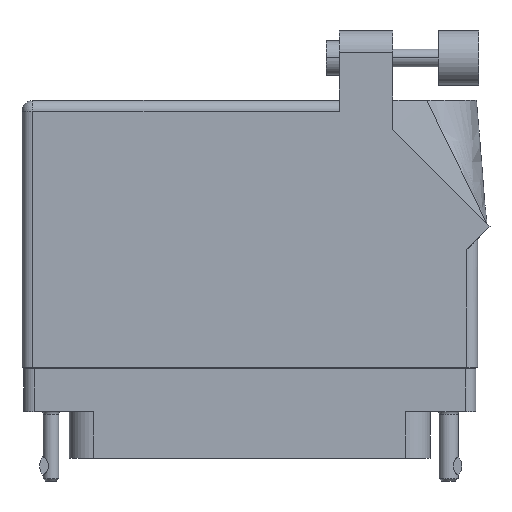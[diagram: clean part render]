
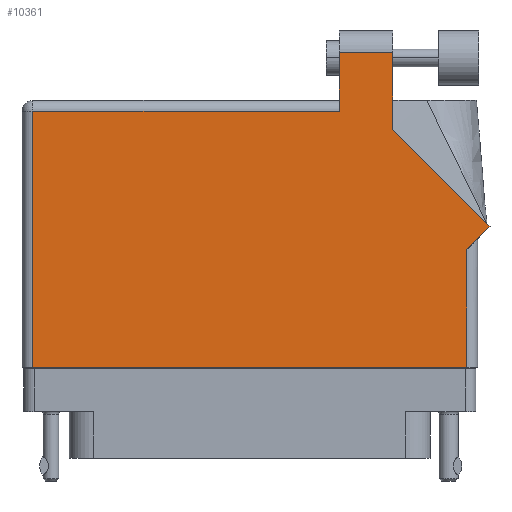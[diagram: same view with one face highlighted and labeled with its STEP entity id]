
A CAD part, front view. The second image highlights one B-rep face of the part: STEP entity #10361.
In plain terms, the highlighted face is planar.
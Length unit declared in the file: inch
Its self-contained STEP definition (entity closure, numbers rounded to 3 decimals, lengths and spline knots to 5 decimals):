
#507 = DIRECTION ( 'NONE',  ( 0., 1., 0. ) ) ;
#3400 = CARTESIAN_POINT ( 'NONE',  ( 1.306, 0.637, 0.455 ) ) ;
#3542 = VERTEX_POINT ( 'NONE', #5887 ) ;
#3811 = ORIENTED_EDGE ( 'NONE', *, *, #17329, .T. ) ;
#4860 = VECTOR ( 'NONE', #46146, 39.37008 ) ;
#5770 = ORIENTED_EDGE ( 'NONE', *, *, #61104, .T. ) ;
#5887 = CARTESIAN_POINT ( 'NONE',  ( 1.37671, 0.70771, 0.455 ) ) ;
#7554 = DIRECTION ( 'NONE',  ( 0., 0., -1. ) ) ;
#8658 = EDGE_LOOP ( 'NONE', ( #59539, #56673, #15471, #14280, #3811, #14995, #5770, #11784, #46687 ) ) ;
#10133 = LINE ( 'NONE', #57187, #55850 ) ;
#10361 = ADVANCED_FACE ( 'NONE', ( #16559 ), #35436, .F. ) ;
#11784 = ORIENTED_EDGE ( 'NONE', *, *, #49289, .T. ) ;
#14280 = ORIENTED_EDGE ( 'NONE', *, *, #25495, .T. ) ;
#14977 = AXIS2_PLACEMENT_3D ( 'NONE', #21819, #7554, #22240 ) ;
#14995 = ORIENTED_EDGE ( 'NONE', *, *, #37256, .T. ) ;
#15471 = ORIENTED_EDGE ( 'NONE', *, *, #34756, .T. ) ;
#16348 = DIRECTION ( 'NONE',  ( 1., 0., 0. ) ) ;
#16489 = VECTOR ( 'NONE', #59213, 39.37008 ) ;
#16559 = FACE_OUTER_BOUND ( 'NONE', #8658, .T. ) ;
#16572 = LINE ( 'NONE', #45083, #37260 ) ;
#16948 = CARTESIAN_POINT ( 'NONE',  ( 0.513, 1.705, 0.455 ) ) ;
#17329 = EDGE_CURVE ( 'NONE', #31396, #21033, #19677, .T. ) ;
#19677 = LINE ( 'NONE', #25045, #28486 ) ;
#21033 = VERTEX_POINT ( 'NONE', #59334 ) ;
#21819 = CARTESIAN_POINT ( 'NONE',  ( -1.306, 1.43, 0.455 ) ) ;
#21882 = VERTEX_POINT ( 'NONE', #48684 ) ;
#22240 = DIRECTION ( 'NONE',  ( -1., 0., 0. ) ) ;
#23289 = VERTEX_POINT ( 'NONE', #16948 ) ;
#23631 = EDGE_CURVE ( 'NONE', #3542, #53780, #16572, .T. ) ;
#25045 = CARTESIAN_POINT ( 'NONE',  ( -1.244, -0.1, 0.455 ) ) ;
#25495 = EDGE_CURVE ( 'NONE', #28730, #31396, #47323, .T. ) ;
#25578 = DIRECTION ( 'NONE',  ( -1., 0., 0. ) ) ;
#25584 = CARTESIAN_POINT ( 'NONE',  ( 0.513, 1.368, 0.455 ) ) ;
#26626 = LINE ( 'NONE', #34705, #42022 ) ;
#27619 = VERTEX_POINT ( 'NONE', #56955 ) ;
#28486 = VECTOR ( 'NONE', #39075, 39.37008 ) ;
#28730 = VERTEX_POINT ( 'NONE', #25584 ) ;
#30913 = LINE ( 'NONE', #33974, #35332 ) ;
#31396 = VERTEX_POINT ( 'NONE', #58039 ) ;
#33974 = CARTESIAN_POINT ( 'NONE',  ( 1.244, 0.637, 0.455 ) ) ;
#33987 = VERTEX_POINT ( 'NONE', #48193 ) ;
#34705 = CARTESIAN_POINT ( 'NONE',  ( -1.306, -0.1, 0.455 ) ) ;
#34756 = EDGE_CURVE ( 'NONE', #23289, #28730, #57760, .T. ) ;
#35332 = VECTOR ( 'NONE', #52729, 39.37008 ) ;
#35436 = PLANE ( 'NONE',  #14977 ) ;
#37256 = EDGE_CURVE ( 'NONE', #21033, #33987, #26626, .T. ) ;
#37260 = VECTOR ( 'NONE', #49786, 39.37008 ) ;
#39075 = DIRECTION ( 'NONE',  ( 0., -1., 0. ) ) ;
#40705 = VECTOR ( 'NONE', #25578, 39.37008 ) ;
#40854 = CARTESIAN_POINT ( 'NONE',  ( 0.513, 1.43, 0.455 ) ) ;
#41080 = CARTESIAN_POINT ( 'NONE',  ( 0.513, 1.705, 0.455 ) ) ;
#42022 = VECTOR ( 'NONE', #16348, 39.37008 ) ;
#45083 = CARTESIAN_POINT ( 'NONE',  ( 1.37671, 0.70771, 0.455 ) ) ;
#45819 = DIRECTION ( 'NONE',  ( -1., 0., 0. ) ) ;
#46146 = DIRECTION ( 'NONE',  ( 0.707, 0.707, 0. ) ) ;
#46687 = ORIENTED_EDGE ( 'NONE', *, *, #23631, .T. ) ;
#46973 = VECTOR ( 'NONE', #45819, 39.37008 ) ;
#47036 = LINE ( 'NONE', #41080, #46973 ) ;
#47323 = LINE ( 'NONE', #54361, #40705 ) ;
#48193 = CARTESIAN_POINT ( 'NONE',  ( 1.244, -0.1, 0.455 ) ) ;
#48612 = EDGE_CURVE ( 'NONE', #53780, #27619, #10133, .T. ) ;
#48684 = CARTESIAN_POINT ( 'NONE',  ( 1.244, 0.575, 0.455 ) ) ;
#49289 = EDGE_CURVE ( 'NONE', #21882, #3542, #50600, .T. ) ;
#49786 = DIRECTION ( 'NONE',  ( -0.707, 0.707, 0. ) ) ;
#50073 = CARTESIAN_POINT ( 'NONE',  ( 0.82, 1.26442, 0.455 ) ) ;
#50600 = LINE ( 'NONE', #3400, #4860 ) ;
#52729 = DIRECTION ( 'NONE',  ( 0., 1., 0. ) ) ;
#53780 = VERTEX_POINT ( 'NONE', #50073 ) ;
#54361 = CARTESIAN_POINT ( 'NONE',  ( -1.306, 1.368, 0.455 ) ) ;
#55850 = VECTOR ( 'NONE', #507, 39.37008 ) ;
#56673 = ORIENTED_EDGE ( 'NONE', *, *, #59417, .T. ) ;
#56955 = CARTESIAN_POINT ( 'NONE',  ( 0.82, 1.705, 0.455 ) ) ;
#57187 = CARTESIAN_POINT ( 'NONE',  ( 0.82, 1.26442, 0.455 ) ) ;
#57760 = LINE ( 'NONE', #40854, #16489 ) ;
#58039 = CARTESIAN_POINT ( 'NONE',  ( -1.244, 1.368, 0.455 ) ) ;
#59213 = DIRECTION ( 'NONE',  ( 0., -1., 0. ) ) ;
#59334 = CARTESIAN_POINT ( 'NONE',  ( -1.244, -0.1, 0.455 ) ) ;
#59417 = EDGE_CURVE ( 'NONE', #27619, #23289, #47036, .T. ) ;
#59539 = ORIENTED_EDGE ( 'NONE', *, *, #48612, .T. ) ;
#61104 = EDGE_CURVE ( 'NONE', #33987, #21882, #30913, .T. ) ;
